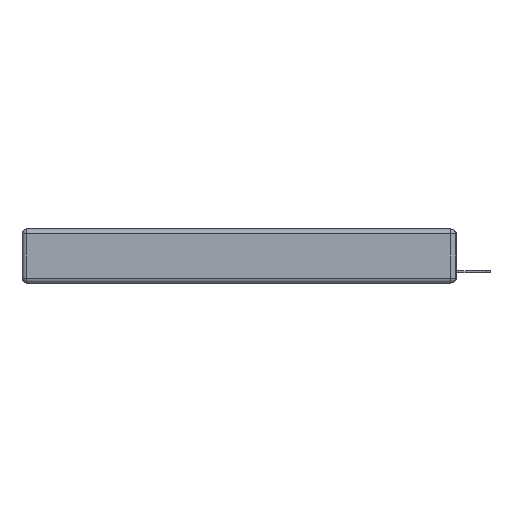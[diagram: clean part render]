
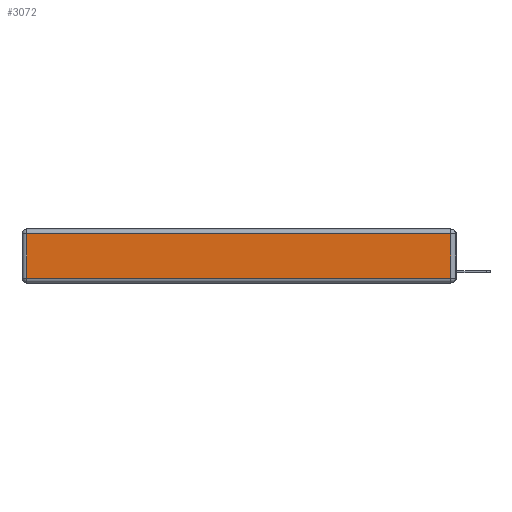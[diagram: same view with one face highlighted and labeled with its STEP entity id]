
A CAD part, left-side view. The second image highlights one B-rep face of the part: STEP entity #3072.
In plain terms, the highlighted planar face has unit normal (-1, 0, 0).
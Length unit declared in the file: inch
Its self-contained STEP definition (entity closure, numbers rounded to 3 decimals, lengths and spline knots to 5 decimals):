
#263 = DIRECTION ( 'NONE',  ( 0., 0., 1. ) ) ;
#441 = LINE ( 'NONE', #3325, #12831 ) ;
#1293 = CARTESIAN_POINT ( 'NONE',  ( 0., 2.75, -0.03 ) ) ;
#2911 = CARTESIAN_POINT ( 'NONE',  ( 0., 0., -0.343 ) ) ;
#3072 = ADVANCED_FACE ( 'NONE', ( #10935 ), #4776, .T. ) ;
#3121 = ORIENTED_EDGE ( 'NONE', *, *, #15368, .T. ) ;
#3325 = CARTESIAN_POINT ( 'NONE',  ( 0., 0., -0.313 ) ) ;
#3426 = CARTESIAN_POINT ( 'NONE',  ( 0., 0.03, -0.343 ) ) ;
#4776 = PLANE ( 'NONE',  #5537 ) ;
#5001 = LINE ( 'NONE', #3426, #5022 ) ;
#5022 = VECTOR ( 'NONE', #263, 39.37008 ) ;
#5105 = LINE ( 'NONE', #11167, #15711 ) ;
#5537 = AXIS2_PLACEMENT_3D ( 'NONE', #2911, #7752, #6380 ) ;
#6137 = EDGE_CURVE ( 'NONE', #13062, #16897, #14877, .T. ) ;
#6380 = DIRECTION ( 'NONE',  ( 0., 0., 1. ) ) ;
#7752 = DIRECTION ( 'NONE',  ( -1., 0., 0. ) ) ;
#8135 = EDGE_CURVE ( 'NONE', #16897, #16561, #5105, .T. ) ;
#9746 = ORIENTED_EDGE ( 'NONE', *, *, #6137, .T. ) ;
#9907 = EDGE_CURVE ( 'NONE', #16561, #11035, #441, .T. ) ;
#10395 = ORIENTED_EDGE ( 'NONE', *, *, #8135, .T. ) ;
#10935 = FACE_OUTER_BOUND ( 'NONE', #16934, .T. ) ;
#11035 = VERTEX_POINT ( 'NONE', #14270 ) ;
#11167 = CARTESIAN_POINT ( 'NONE',  ( 0., 2.72, -0.343 ) ) ;
#11377 = CARTESIAN_POINT ( 'NONE',  ( 0., 2.72, -0.313 ) ) ;
#11902 = DIRECTION ( 'NONE',  ( 0., 1., 0. ) ) ;
#12550 = DIRECTION ( 'NONE',  ( 0., -1., 0. ) ) ;
#12831 = VECTOR ( 'NONE', #12550, 39.37008 ) ;
#13026 = CARTESIAN_POINT ( 'NONE',  ( 0., 2.72, -0.03 ) ) ;
#13062 = VERTEX_POINT ( 'NONE', #17624 ) ;
#14270 = CARTESIAN_POINT ( 'NONE',  ( 0., 0.03, -0.313 ) ) ;
#14877 = LINE ( 'NONE', #1293, #15952 ) ;
#15368 = EDGE_CURVE ( 'NONE', #11035, #13062, #5001, .T. ) ;
#15439 = ORIENTED_EDGE ( 'NONE', *, *, #9907, .T. ) ;
#15711 = VECTOR ( 'NONE', #18863, 39.37008 ) ;
#15952 = VECTOR ( 'NONE', #11902, 39.37008 ) ;
#16561 = VERTEX_POINT ( 'NONE', #11377 ) ;
#16897 = VERTEX_POINT ( 'NONE', #13026 ) ;
#16934 = EDGE_LOOP ( 'NONE', ( #15439, #3121, #9746, #10395 ) ) ;
#17624 = CARTESIAN_POINT ( 'NONE',  ( 0., 0.03, -0.03 ) ) ;
#18863 = DIRECTION ( 'NONE',  ( 0., 0., -1. ) ) ;
